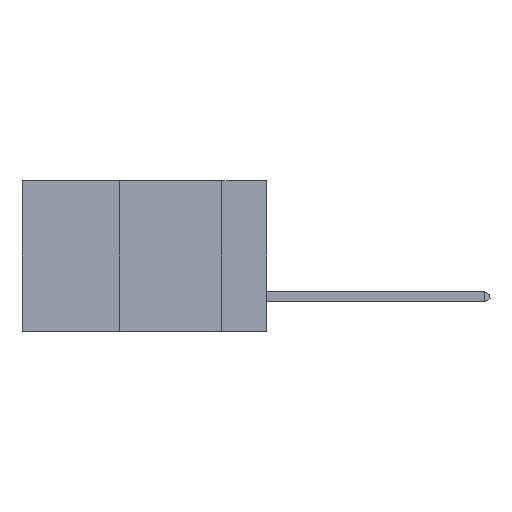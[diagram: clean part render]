
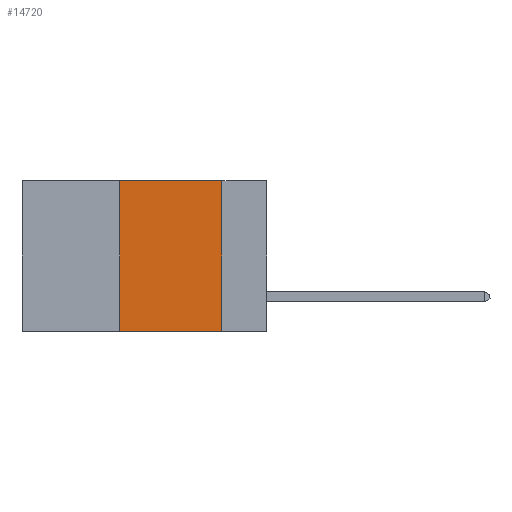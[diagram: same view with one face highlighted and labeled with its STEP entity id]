
A CAD part, left-side view. The second image highlights one B-rep face of the part: STEP entity #14720.
In plain terms, the highlighted planar face has unit normal (-1, 0, 0).
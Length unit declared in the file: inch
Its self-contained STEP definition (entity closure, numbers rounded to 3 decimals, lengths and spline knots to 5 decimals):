
#769 = VERTEX_POINT ( 'NONE', #18231 ) ;
#798 = LINE ( 'NONE', #5885, #15183 ) ;
#1637 = VECTOR ( 'NONE', #10727, 39.37008 ) ;
#2322 = VECTOR ( 'NONE', #8365, 39.37008 ) ;
#2888 = AXIS2_PLACEMENT_3D ( 'NONE', #18347, #6254, #20403 ) ;
#2912 = DIRECTION ( 'NONE',  ( 0., 0., -1. ) ) ;
#3585 = VERTEX_POINT ( 'NONE', #11304 ) ;
#4301 = EDGE_CURVE ( 'NONE', #3585, #769, #798, .T. ) ;
#5885 = CARTESIAN_POINT ( 'NONE',  ( 0., 0.36, 0. ) ) ;
#6254 = DIRECTION ( 'NONE',  ( 1., 0., 0. ) ) ;
#7119 = FACE_OUTER_BOUND ( 'NONE', #20661, .T. ) ;
#7795 = LINE ( 'NONE', #22769, #1637 ) ;
#7920 = ORIENTED_EDGE ( 'NONE', *, *, #9280, .F. ) ;
#8365 = DIRECTION ( 'NONE',  ( 0., -1., 0. ) ) ;
#9280 = EDGE_CURVE ( 'NONE', #21787, #23931, #17460, .T. ) ;
#10727 = DIRECTION ( 'NONE',  ( 0., -1., 0. ) ) ;
#11304 = CARTESIAN_POINT ( 'NONE',  ( 0., 0.36, -0.37 ) ) ;
#11617 = CARTESIAN_POINT ( 'NONE',  ( 0., 0.11, 0. ) ) ;
#13208 = LINE ( 'NONE', #20384, #2322 ) ;
#14720 = ADVANCED_FACE ( 'NONE', ( #7119 ), #16300, .F. ) ;
#15102 = CARTESIAN_POINT ( 'NONE',  ( 0., 0.11, 0. ) ) ;
#15183 = VECTOR ( 'NONE', #23667, 39.37008 ) ;
#16105 = CARTESIAN_POINT ( 'NONE',  ( 0., 0.11, -0.37 ) ) ;
#16300 = PLANE ( 'NONE',  #2888 ) ;
#17408 = ORIENTED_EDGE ( 'NONE', *, *, #19430, .T. ) ;
#17460 = LINE ( 'NONE', #15102, #25507 ) ;
#18231 = CARTESIAN_POINT ( 'NONE',  ( 0., 0.36, 0. ) ) ;
#18347 = CARTESIAN_POINT ( 'NONE',  ( 0., 0.6, 0. ) ) ;
#19430 = EDGE_CURVE ( 'NONE', #3585, #23931, #7795, .T. ) ;
#20384 = CARTESIAN_POINT ( 'NONE',  ( 0., 0.6, 0. ) ) ;
#20403 = DIRECTION ( 'NONE',  ( 0., 0., -1. ) ) ;
#20661 = EDGE_LOOP ( 'NONE', ( #7920, #23347, #22104, #17408 ) ) ;
#21787 = VERTEX_POINT ( 'NONE', #11617 ) ;
#22104 = ORIENTED_EDGE ( 'NONE', *, *, #4301, .F. ) ;
#22769 = CARTESIAN_POINT ( 'NONE',  ( 0., 0.6, -0.37 ) ) ;
#23347 = ORIENTED_EDGE ( 'NONE', *, *, #24008, .F. ) ;
#23667 = DIRECTION ( 'NONE',  ( 0., 0., 1. ) ) ;
#23931 = VERTEX_POINT ( 'NONE', #16105 ) ;
#24008 = EDGE_CURVE ( 'NONE', #769, #21787, #13208, .T. ) ;
#25507 = VECTOR ( 'NONE', #2912, 39.37008 ) ;
